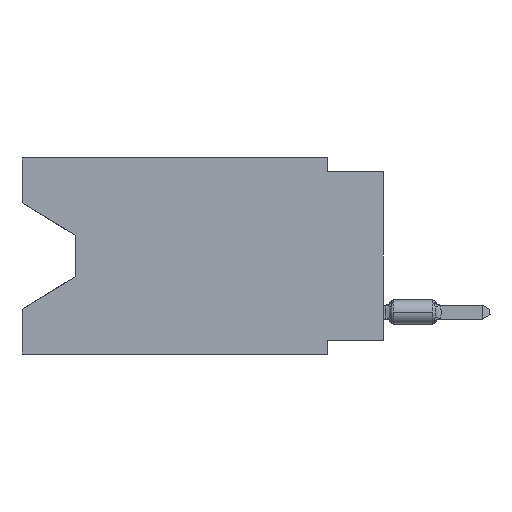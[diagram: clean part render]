
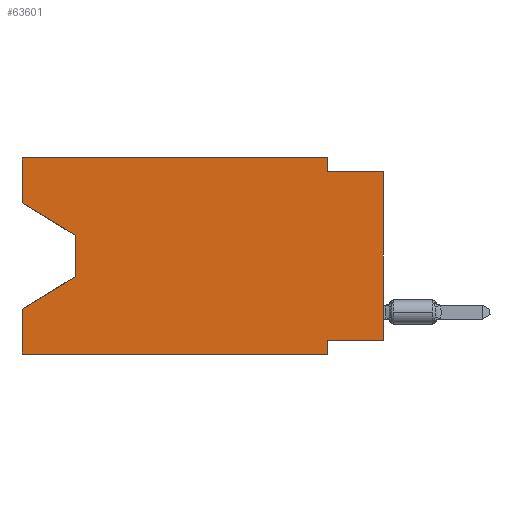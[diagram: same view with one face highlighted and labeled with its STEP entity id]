
A CAD part, left-side view. The second image highlights one B-rep face of the part: STEP entity #63601.
In plain terms, the highlighted planar face has unit normal (-1, 0, 0).
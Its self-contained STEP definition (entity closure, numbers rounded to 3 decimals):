
#90 = DIRECTION ( 'NONE',  ( 0., 0.855, -0.519 ) ) ;
#178 = VECTOR ( 'NONE', #90, 1000. ) ;
#528 = LINE ( 'NONE', #26103, #28309 ) ;
#544 = VECTOR ( 'NONE', #74202, 1000. ) ;
#2067 = EDGE_LOOP ( 'NONE', ( #15302, #11450, #62091, #6105, #21370, #50900, #12609, #55887, #19570, #7464, #35501, #22315 ) ) ;
#2569 = VERTEX_POINT ( 'NONE', #41828 ) ;
#2658 = VERTEX_POINT ( 'NONE', #48951 ) ;
#5517 = DIRECTION ( 'NONE',  ( 0., -0.855, -0.519 ) ) ;
#6105 = ORIENTED_EDGE ( 'NONE', *, *, #42150, .F. ) ;
#6548 = EDGE_CURVE ( 'NONE', #19967, #2658, #27632, .T. ) ;
#7464 = ORIENTED_EDGE ( 'NONE', *, *, #81196, .F. ) ;
#9111 = CARTESIAN_POINT ( 'NONE',  ( 0., 13.97, -3.505 ) ) ;
#9156 = LINE ( 'NONE', #42246, #27721 ) ;
#10477 = DIRECTION ( 'NONE',  ( 0., 0., 1. ) ) ;
#11323 = CARTESIAN_POINT ( 'NONE',  ( 0., 16.383, -6.852 ) ) ;
#11450 = ORIENTED_EDGE ( 'NONE', *, *, #6548, .T. ) ;
#11973 = VERTEX_POINT ( 'NONE', #25485 ) ;
#12492 = VERTEX_POINT ( 'NONE', #59339 ) ;
#12609 = ORIENTED_EDGE ( 'NONE', *, *, #46242, .F. ) ;
#13275 = DIRECTION ( 'NONE',  ( 0., 0., 1. ) ) ;
#15302 = ORIENTED_EDGE ( 'NONE', *, *, #35888, .T. ) ;
#15394 = EDGE_CURVE ( 'NONE', #25273, #45301, #24890, .T. ) ;
#16301 = LINE ( 'NONE', #48592, #544 ) ;
#16413 = VERTEX_POINT ( 'NONE', #61430 ) ;
#16713 = VECTOR ( 'NONE', #20004, 1000. ) ;
#18897 = VECTOR ( 'NONE', #80766, 1000. ) ;
#19570 = ORIENTED_EDGE ( 'NONE', *, *, #80841, .F. ) ;
#19591 = CARTESIAN_POINT ( 'NONE',  ( 0., 2.54, 0. ) ) ;
#19967 = VERTEX_POINT ( 'NONE', #9111 ) ;
#20004 = DIRECTION ( 'NONE',  ( 0., 0., -1. ) ) ;
#21370 = ORIENTED_EDGE ( 'NONE', *, *, #15394, .T. ) ;
#22315 = ORIENTED_EDGE ( 'NONE', *, *, #61603, .F. ) ;
#22827 = VECTOR ( 'NONE', #13275, 1000. ) ;
#22849 = LINE ( 'NONE', #29537, #18897 ) ;
#23484 = LINE ( 'NONE', #66321, #45797 ) ;
#24890 = LINE ( 'NONE', #68114, #27194 ) ;
#24955 = LINE ( 'NONE', #61902, #67793 ) ;
#25273 = VERTEX_POINT ( 'NONE', #75826 ) ;
#25485 = CARTESIAN_POINT ( 'NONE',  ( 0., 16.383, 0. ) ) ;
#25624 = DIRECTION ( 'NONE',  ( 1., 0., 0. ) ) ;
#26103 = CARTESIAN_POINT ( 'NONE',  ( 0., 0., -8.255 ) ) ;
#26446 = CARTESIAN_POINT ( 'NONE',  ( 0., 2.54, -8.255 ) ) ;
#27194 = VECTOR ( 'NONE', #76092, 1000. ) ;
#27632 = LINE ( 'NONE', #72119, #71609 ) ;
#27721 = VECTOR ( 'NONE', #41024, 1000. ) ;
#28309 = VECTOR ( 'NONE', #31979, 1000. ) ;
#29537 = CARTESIAN_POINT ( 'NONE',  ( 0., 2.54, -8.89 ) ) ;
#29539 = CARTESIAN_POINT ( 'NONE',  ( 0., 16.383, -2.038 ) ) ;
#31079 = EDGE_CURVE ( 'NONE', #2569, #62458, #24955, .T. ) ;
#31945 = EDGE_CURVE ( 'NONE', #11973, #16413, #9156, .T. ) ;
#31979 = DIRECTION ( 'NONE',  ( 0., 1., 0. ) ) ;
#35501 = ORIENTED_EDGE ( 'NONE', *, *, #31945, .F. ) ;
#35888 = EDGE_CURVE ( 'NONE', #61578, #19967, #74461, .T. ) ;
#37418 = EDGE_CURVE ( 'NONE', #2658, #43407, #82373, .T. ) ;
#39678 = LINE ( 'NONE', #71588, #22827 ) ;
#41024 = DIRECTION ( 'NONE',  ( 0., -1., 0. ) ) ;
#41298 = EDGE_CURVE ( 'NONE', #63587, #45301, #22849, .T. ) ;
#41828 = CARTESIAN_POINT ( 'NONE',  ( 0., 0., -8.255 ) ) ;
#42150 = EDGE_CURVE ( 'NONE', #25273, #43407, #23484, .T. ) ;
#42246 = CARTESIAN_POINT ( 'NONE',  ( 0., 16.383, 0. ) ) ;
#42570 = DIRECTION ( 'NONE',  ( 0., 0., 1. ) ) ;
#43407 = VERTEX_POINT ( 'NONE', #11323 ) ;
#44172 = VECTOR ( 'NONE', #5517, 1000. ) ;
#45301 = VERTEX_POINT ( 'NONE', #67885 ) ;
#45325 = DIRECTION ( 'NONE',  ( 0., 0., -1. ) ) ;
#45797 = VECTOR ( 'NONE', #10477, 1000. ) ;
#46242 = EDGE_CURVE ( 'NONE', #2569, #63587, #528, .T. ) ;
#48592 = CARTESIAN_POINT ( 'NONE',  ( 0., 0., -0.635 ) ) ;
#48951 = CARTESIAN_POINT ( 'NONE',  ( 0., 13.97, -5.385 ) ) ;
#50448 = CARTESIAN_POINT ( 'NONE',  ( 0., 13.97, -5.385 ) ) ;
#50900 = ORIENTED_EDGE ( 'NONE', *, *, #41298, .F. ) ;
#55887 = ORIENTED_EDGE ( 'NONE', *, *, #31079, .T. ) ;
#57513 = FACE_OUTER_BOUND ( 'NONE', #2067, .T. ) ;
#59339 = CARTESIAN_POINT ( 'NONE',  ( 0., 2.54, -0.635 ) ) ;
#61430 = CARTESIAN_POINT ( 'NONE',  ( 0., 2.54, 0. ) ) ;
#61578 = VERTEX_POINT ( 'NONE', #75417 ) ;
#61603 = EDGE_CURVE ( 'NONE', #61578, #11973, #39678, .T. ) ;
#61902 = CARTESIAN_POINT ( 'NONE',  ( 0., 0., 0. ) ) ;
#62091 = ORIENTED_EDGE ( 'NONE', *, *, #37418, .T. ) ;
#62458 = VERTEX_POINT ( 'NONE', #72107 ) ;
#63587 = VERTEX_POINT ( 'NONE', #26446 ) ;
#63601 = ADVANCED_FACE ( 'NONE', ( #57513 ), #64220, .F. ) ;
#64220 = PLANE ( 'NONE',  #73745 ) ;
#66321 = CARTESIAN_POINT ( 'NONE',  ( 0., 16.383, 0. ) ) ;
#67793 = VECTOR ( 'NONE', #42570, 1000. ) ;
#67885 = CARTESIAN_POINT ( 'NONE',  ( 0., 2.54, -8.89 ) ) ;
#68114 = CARTESIAN_POINT ( 'NONE',  ( 0., 16.383, -8.89 ) ) ;
#70525 = CARTESIAN_POINT ( 'NONE',  ( 0., 16.383, 0. ) ) ;
#71588 = CARTESIAN_POINT ( 'NONE',  ( 0., 16.383, 0. ) ) ;
#71609 = VECTOR ( 'NONE', #78837, 1000. ) ;
#72107 = CARTESIAN_POINT ( 'NONE',  ( 0., 0., -0.635 ) ) ;
#72119 = CARTESIAN_POINT ( 'NONE',  ( 0., 13.97, -3.505 ) ) ;
#73745 = AXIS2_PLACEMENT_3D ( 'NONE', #70525, #25624, #45325 ) ;
#74202 = DIRECTION ( 'NONE',  ( 0., -1., 0. ) ) ;
#74461 = LINE ( 'NONE', #29539, #44172 ) ;
#75417 = CARTESIAN_POINT ( 'NONE',  ( 0., 16.383, -2.038 ) ) ;
#75826 = CARTESIAN_POINT ( 'NONE',  ( 0., 16.383, -8.89 ) ) ;
#76092 = DIRECTION ( 'NONE',  ( 0., -1., 0. ) ) ;
#77105 = LINE ( 'NONE', #19591, #16713 ) ;
#78837 = DIRECTION ( 'NONE',  ( 0., 0., -1. ) ) ;
#80766 = DIRECTION ( 'NONE',  ( 0., 0., -1. ) ) ;
#80841 = EDGE_CURVE ( 'NONE', #12492, #62458, #16301, .T. ) ;
#81196 = EDGE_CURVE ( 'NONE', #16413, #12492, #77105, .T. ) ;
#82373 = LINE ( 'NONE', #50448, #178 ) ;
